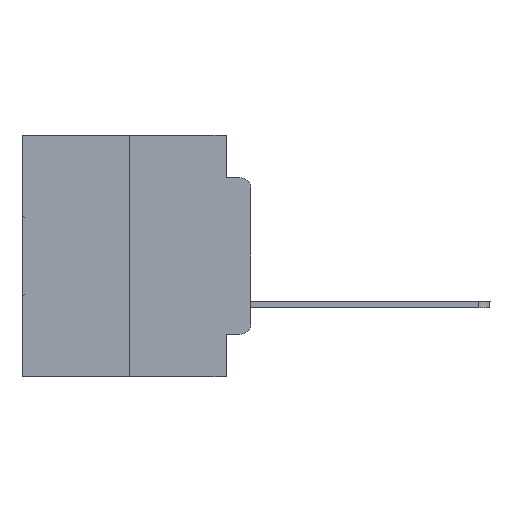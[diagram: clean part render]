
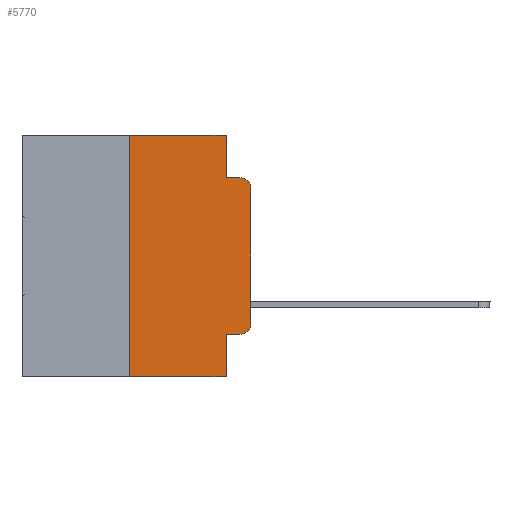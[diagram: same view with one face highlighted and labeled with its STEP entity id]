
A CAD part, left-side view. The second image highlights one B-rep face of the part: STEP entity #5770.
In plain terms, the highlighted planar face has unit normal (-1, 0, 0).
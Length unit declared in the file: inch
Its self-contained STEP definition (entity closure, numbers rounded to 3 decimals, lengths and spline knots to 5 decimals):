
#875 = VERTEX_POINT ( 'NONE', #2707 ) ;
#984 = PLANE ( 'NONE',  #16287 ) ;
#1629 = DIRECTION ( 'NONE',  ( 0., 0., -1. ) ) ;
#2282 = CARTESIAN_POINT ( 'NONE',  ( 0., 0.051, 0. ) ) ;
#2707 = CARTESIAN_POINT ( 'NONE',  ( 0., 0.02, -0.4115 ) ) ;
#3550 = DIRECTION ( 'NONE',  ( 1., 0., 0. ) ) ;
#3788 = DIRECTION ( 'NONE',  ( 0., 0., -1. ) ) ;
#3964 = VECTOR ( 'NONE', #22808, 39.37008 ) ;
#4051 = EDGE_CURVE ( 'NONE', #875, #9134, #25567, .T. ) ;
#4213 = DIRECTION ( 'NONE',  ( 0., 0., 1. ) ) ;
#4724 = VERTEX_POINT ( 'NONE', #5363 ) ;
#5059 = VERTEX_POINT ( 'NONE', #25319 ) ;
#5260 = DIRECTION ( 'NONE',  ( 0., -1., 0. ) ) ;
#5363 = CARTESIAN_POINT ( 'NONE',  ( 0., 0.25, -0.5 ) ) ;
#5770 = ADVANCED_FACE ( 'NONE', ( #7502 ), #984, .F. ) ;
#6059 = VECTOR ( 'NONE', #10592, 39.37008 ) ;
#6101 = DIRECTION ( 'NONE',  ( 0., -1., 0. ) ) ;
#6313 = ORIENTED_EDGE ( 'NONE', *, *, #31419, .T. ) ;
#6474 = LINE ( 'NONE', #20865, #6059 ) ;
#6532 = CARTESIAN_POINT ( 'NONE',  ( 0., 0.02, -0.0885 ) ) ;
#7502 = FACE_OUTER_BOUND ( 'NONE', #20704, .T. ) ;
#8198 = CARTESIAN_POINT ( 'NONE',  ( 0., 0.473, 0. ) ) ;
#8390 = VECTOR ( 'NONE', #19954, 39.37008 ) ;
#8585 = ORIENTED_EDGE ( 'NONE', *, *, #32065, .T. ) ;
#8805 = DIRECTION ( 'NONE',  ( -1., 0., 0. ) ) ;
#8812 = VERTEX_POINT ( 'NONE', #18895 ) ;
#8860 = ORIENTED_EDGE ( 'NONE', *, *, #4051, .T. ) ;
#9134 = VERTEX_POINT ( 'NONE', #31457 ) ;
#9195 = VERTEX_POINT ( 'NONE', #6532 ) ;
#10108 = ORIENTED_EDGE ( 'NONE', *, *, #28191, .F. ) ;
#10592 = DIRECTION ( 'NONE',  ( 0., 0., 1. ) ) ;
#10970 = DIRECTION ( 'NONE',  ( 0., 0., -1. ) ) ;
#10994 = ORIENTED_EDGE ( 'NONE', *, *, #17733, .T. ) ;
#11085 = DIRECTION ( 'NONE',  ( 0., 0., -1. ) ) ;
#13110 = VECTOR ( 'NONE', #6101, 39.37008 ) ;
#13476 = CARTESIAN_POINT ( 'NONE',  ( 0., 0.473, 0. ) ) ;
#14235 = EDGE_CURVE ( 'NONE', #25549, #9195, #15572, .T. ) ;
#14244 = LINE ( 'NONE', #27791, #3964 ) ;
#14378 = AXIS2_PLACEMENT_3D ( 'NONE', #24402, #8805, #1629 ) ;
#15492 = LINE ( 'NONE', #8198, #13110 ) ;
#15572 = LINE ( 'NONE', #21914, #31773 ) ;
#15776 = VERTEX_POINT ( 'NONE', #16247 ) ;
#16053 = CARTESIAN_POINT ( 'NONE',  ( 0., 0.02, -0.1085 ) ) ;
#16217 = VERTEX_POINT ( 'NONE', #30487 ) ;
#16247 = CARTESIAN_POINT ( 'NONE',  ( 0., 0.051, 0. ) ) ;
#16261 = VECTOR ( 'NONE', #4213, 39.37008 ) ;
#16287 = AXIS2_PLACEMENT_3D ( 'NONE', #13476, #3550, #3788 ) ;
#16740 = VECTOR ( 'NONE', #5260, 39.37008 ) ;
#17733 = EDGE_CURVE ( 'NONE', #17871, #875, #14244, .T. ) ;
#17871 = VERTEX_POINT ( 'NONE', #22550 ) ;
#17892 = ORIENTED_EDGE ( 'NONE', *, *, #22989, .F. ) ;
#18895 = CARTESIAN_POINT ( 'NONE',  ( 0., 0., -0.1085 ) ) ;
#19479 = CIRCLE ( 'NONE', #28444, 0.02 ) ;
#19954 = DIRECTION ( 'NONE',  ( 0., 0., -1. ) ) ;
#20704 = EDGE_LOOP ( 'NONE', ( #6313, #24012, #21835, #31407, #31728, #17892, #8585, #10108, #10994, #8860 ) ) ;
#20865 = CARTESIAN_POINT ( 'NONE',  ( 0., 0., 0. ) ) ;
#21835 = ORIENTED_EDGE ( 'NONE', *, *, #14235, .F. ) ;
#21909 = LINE ( 'NONE', #32678, #16740 ) ;
#21914 = CARTESIAN_POINT ( 'NONE',  ( 0., 0.051, -0.0885 ) ) ;
#22257 = LINE ( 'NONE', #2282, #8390 ) ;
#22550 = CARTESIAN_POINT ( 'NONE',  ( 0., 0.051, -0.4115 ) ) ;
#22808 = DIRECTION ( 'NONE',  ( 0., -1., 0. ) ) ;
#22989 = EDGE_CURVE ( 'NONE', #4724, #5059, #30471, .T. ) ;
#23801 = DIRECTION ( 'NONE',  ( -1., 0., 0. ) ) ;
#24012 = ORIENTED_EDGE ( 'NONE', *, *, #32357, .T. ) ;
#24402 = CARTESIAN_POINT ( 'NONE',  ( 0., 0.02, -0.3915 ) ) ;
#24452 = DIRECTION ( 'NONE',  ( 0., -1., 0. ) ) ;
#24540 = CARTESIAN_POINT ( 'NONE',  ( 0., 0.25, 0. ) ) ;
#25319 = CARTESIAN_POINT ( 'NONE',  ( 0., 0.25, 0. ) ) ;
#25549 = VERTEX_POINT ( 'NONE', #25819 ) ;
#25567 = CIRCLE ( 'NONE', #14378, 0.02 ) ;
#25797 = LINE ( 'NONE', #26714, #27014 ) ;
#25819 = CARTESIAN_POINT ( 'NONE',  ( 0., 0.051, -0.0885 ) ) ;
#26714 = CARTESIAN_POINT ( 'NONE',  ( 0., 0.051, 0. ) ) ;
#27014 = VECTOR ( 'NONE', #11085, 39.37008 ) ;
#27791 = CARTESIAN_POINT ( 'NONE',  ( 0., 0.051, -0.4115 ) ) ;
#28191 = EDGE_CURVE ( 'NONE', #17871, #16217, #22257, .T. ) ;
#28444 = AXIS2_PLACEMENT_3D ( 'NONE', #16053, #23801, #10970 ) ;
#30471 = LINE ( 'NONE', #24540, #16261 ) ;
#30487 = CARTESIAN_POINT ( 'NONE',  ( 0., 0.051, -0.5 ) ) ;
#31407 = ORIENTED_EDGE ( 'NONE', *, *, #32329, .F. ) ;
#31419 = EDGE_CURVE ( 'NONE', #9134, #8812, #6474, .T. ) ;
#31457 = CARTESIAN_POINT ( 'NONE',  ( 0., 0., -0.3915 ) ) ;
#31728 = ORIENTED_EDGE ( 'NONE', *, *, #32433, .F. ) ;
#31773 = VECTOR ( 'NONE', #24452, 39.37008 ) ;
#32065 = EDGE_CURVE ( 'NONE', #4724, #16217, #21909, .T. ) ;
#32329 = EDGE_CURVE ( 'NONE', #15776, #25549, #25797, .T. ) ;
#32357 = EDGE_CURVE ( 'NONE', #8812, #9195, #19479, .T. ) ;
#32433 = EDGE_CURVE ( 'NONE', #5059, #15776, #15492, .T. ) ;
#32678 = CARTESIAN_POINT ( 'NONE',  ( 0., 0.473, -0.5 ) ) ;
